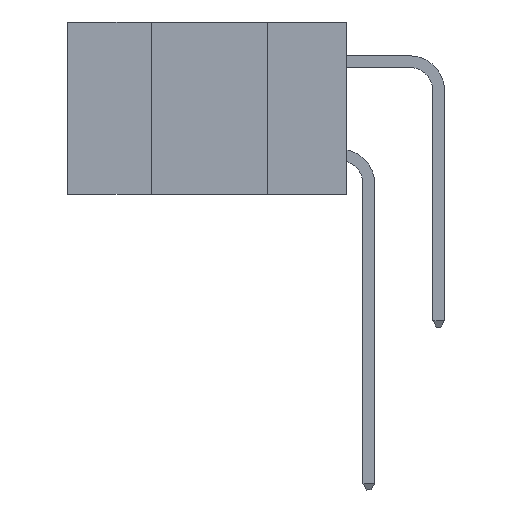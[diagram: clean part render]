
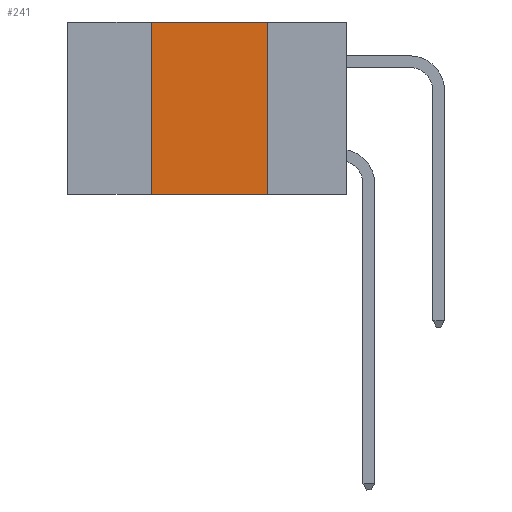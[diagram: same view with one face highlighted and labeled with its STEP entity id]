
A CAD part, left-side view. The second image highlights one B-rep face of the part: STEP entity #241.
In plain terms, the highlighted planar face has unit normal (-1, 0, 0).
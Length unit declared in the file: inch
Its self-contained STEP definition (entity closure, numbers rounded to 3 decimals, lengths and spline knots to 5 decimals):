
#241 = ADVANCED_FACE ( 'NONE', ( #6327 ), #5556, .F. ) ;
#784 = VERTEX_POINT ( 'NONE', #5878 ) ;
#1549 = DIRECTION ( 'NONE',  ( 0., 0., 1. ) ) ;
#1960 = EDGE_CURVE ( 'NONE', #784, #9471, #5156, .T. ) ;
#2009 = VERTEX_POINT ( 'NONE', #2217 ) ;
#2084 = ORIENTED_EDGE ( 'NONE', *, *, #9118, .T. ) ;
#2217 = CARTESIAN_POINT ( 'NONE',  ( 0., 0.17, -0.37 ) ) ;
#2771 = DIRECTION ( 'NONE',  ( 0., -1., 0. ) ) ;
#3012 = EDGE_LOOP ( 'NONE', ( #14210, #4483, #4833, #2084 ) ) ;
#3715 = LINE ( 'NONE', #5790, #12975 ) ;
#3948 = CARTESIAN_POINT ( 'NONE',  ( 0., 0.42, 0. ) ) ;
#4483 = ORIENTED_EDGE ( 'NONE', *, *, #1960, .F. ) ;
#4711 = VECTOR ( 'NONE', #14862, 39.37008 ) ;
#4833 = ORIENTED_EDGE ( 'NONE', *, *, #9891, .F. ) ;
#5156 = LINE ( 'NONE', #10935, #11000 ) ;
#5217 = CARTESIAN_POINT ( 'NONE',  ( 0., 0.6, 0. ) ) ;
#5444 = LINE ( 'NONE', #13752, #4711 ) ;
#5556 = PLANE ( 'NONE',  #9952 ) ;
#5790 = CARTESIAN_POINT ( 'NONE',  ( 0., 0.17, 0. ) ) ;
#5878 = CARTESIAN_POINT ( 'NONE',  ( 0., 0.42, 0. ) ) ;
#6327 = FACE_OUTER_BOUND ( 'NONE', #3012, .T. ) ;
#6339 = DIRECTION ( 'NONE',  ( 1., 0., 0. ) ) ;
#6460 = DIRECTION ( 'NONE',  ( 0., 0., -1. ) ) ;
#9118 = EDGE_CURVE ( 'NONE', #11463, #2009, #5444, .T. ) ;
#9321 = CARTESIAN_POINT ( 'NONE',  ( 0., 0.42, -0.37 ) ) ;
#9471 = VERTEX_POINT ( 'NONE', #14610 ) ;
#9891 = EDGE_CURVE ( 'NONE', #11463, #784, #10522, .T. ) ;
#9952 = AXIS2_PLACEMENT_3D ( 'NONE', #5217, #6339, #6460 ) ;
#10522 = LINE ( 'NONE', #3948, #13564 ) ;
#10935 = CARTESIAN_POINT ( 'NONE',  ( 0., 0.6, 0. ) ) ;
#11000 = VECTOR ( 'NONE', #2771, 39.37008 ) ;
#11440 = EDGE_CURVE ( 'NONE', #9471, #2009, #3715, .T. ) ;
#11463 = VERTEX_POINT ( 'NONE', #9321 ) ;
#12975 = VECTOR ( 'NONE', #14988, 39.37008 ) ;
#13564 = VECTOR ( 'NONE', #1549, 39.37008 ) ;
#13752 = CARTESIAN_POINT ( 'NONE',  ( 0., 0.6, -0.37 ) ) ;
#14210 = ORIENTED_EDGE ( 'NONE', *, *, #11440, .F. ) ;
#14610 = CARTESIAN_POINT ( 'NONE',  ( 0., 0.17, 0. ) ) ;
#14862 = DIRECTION ( 'NONE',  ( 0., -1., 0. ) ) ;
#14988 = DIRECTION ( 'NONE',  ( 0., 0., -1. ) ) ;
